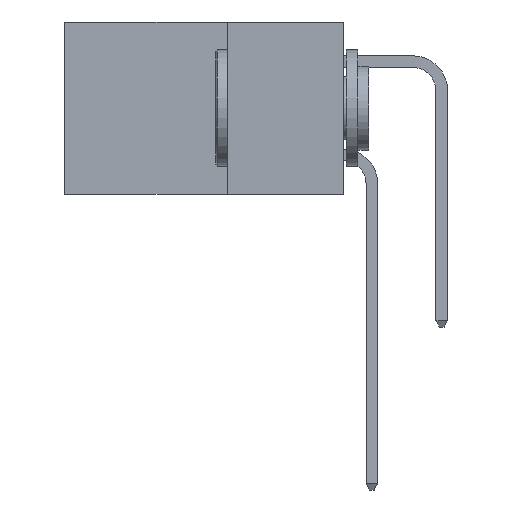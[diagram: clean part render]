
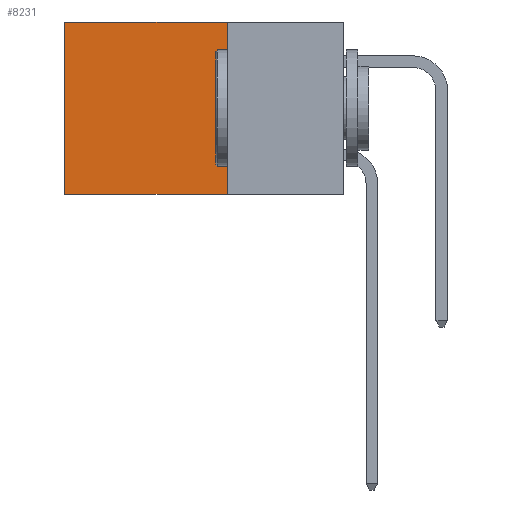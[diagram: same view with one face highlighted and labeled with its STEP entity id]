
A CAD part, left-side view. The second image highlights one B-rep face of the part: STEP entity #8231.
In plain terms, the highlighted planar face has unit normal (-1, 0, 0).
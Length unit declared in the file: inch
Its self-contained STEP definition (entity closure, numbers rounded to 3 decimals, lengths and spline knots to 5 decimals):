
#2493 = VECTOR ( 'NONE', #8146, 39.37008 ) ;
#2675 = EDGE_CURVE ( 'NONE', #8858, #2737, #11368, .T. ) ;
#2737 = VERTEX_POINT ( 'NONE', #3919 ) ;
#3371 = AXIS2_PLACEMENT_3D ( 'NONE', #12109, #11923, #11915 ) ;
#3919 = CARTESIAN_POINT ( 'NONE',  ( 0.2615, 0.6, 0. ) ) ;
#4006 = LINE ( 'NONE', #8329, #12666 ) ;
#4669 = ORIENTED_EDGE ( 'NONE', *, *, #14275, .F. ) ;
#4703 = EDGE_LOOP ( 'NONE', ( #7932, #4669, #14230, #9532 ) ) ;
#4789 = EDGE_CURVE ( 'NONE', #8858, #9702, #7465, .T. ) ;
#4998 = VECTOR ( 'NONE', #6668, 39.37008 ) ;
#5475 = CARTESIAN_POINT ( 'NONE',  ( 0.2615, 0.25, 0. ) ) ;
#5840 = FACE_OUTER_BOUND ( 'NONE', #4703, .T. ) ;
#6668 = DIRECTION ( 'NONE',  ( 0., 1., 0. ) ) ;
#6721 = CARTESIAN_POINT ( 'NONE',  ( 0.2615, 0.25, 0. ) ) ;
#7397 = EDGE_CURVE ( 'NONE', #2737, #14046, #8167, .T. ) ;
#7465 = LINE ( 'NONE', #11857, #9760 ) ;
#7932 = ORIENTED_EDGE ( 'NONE', *, *, #7397, .T. ) ;
#7980 = CARTESIAN_POINT ( 'NONE',  ( 0.2615, 0.6, -0.37 ) ) ;
#8146 = DIRECTION ( 'NONE',  ( 0., 0., -1. ) ) ;
#8167 = LINE ( 'NONE', #7980, #2493 ) ;
#8231 = ADVANCED_FACE ( 'NONE', ( #5840 ), #12163, .F. ) ;
#8278 = DIRECTION ( 'NONE',  ( 0., 1., 0. ) ) ;
#8329 = CARTESIAN_POINT ( 'NONE',  ( 0.2615, 0.25, -0.37 ) ) ;
#8858 = VERTEX_POINT ( 'NONE', #6721 ) ;
#9203 = CARTESIAN_POINT ( 'NONE',  ( 0.2615, 0.25, -0.37 ) ) ;
#9532 = ORIENTED_EDGE ( 'NONE', *, *, #2675, .T. ) ;
#9702 = VERTEX_POINT ( 'NONE', #9203 ) ;
#9760 = VECTOR ( 'NONE', #12223, 39.37008 ) ;
#10356 = CARTESIAN_POINT ( 'NONE',  ( 0.2615, 0.6, -0.37 ) ) ;
#11368 = LINE ( 'NONE', #5475, #4998 ) ;
#11857 = CARTESIAN_POINT ( 'NONE',  ( 0.2615, 0.25, -0.37 ) ) ;
#11915 = DIRECTION ( 'NONE',  ( 0., 0., -1. ) ) ;
#11923 = DIRECTION ( 'NONE',  ( 1., 0., 0. ) ) ;
#12109 = CARTESIAN_POINT ( 'NONE',  ( 0.2615, 0.25, -0.37 ) ) ;
#12163 = PLANE ( 'NONE',  #3371 ) ;
#12223 = DIRECTION ( 'NONE',  ( 0., 0., -1. ) ) ;
#12666 = VECTOR ( 'NONE', #8278, 39.37008 ) ;
#14046 = VERTEX_POINT ( 'NONE', #10356 ) ;
#14230 = ORIENTED_EDGE ( 'NONE', *, *, #4789, .F. ) ;
#14275 = EDGE_CURVE ( 'NONE', #9702, #14046, #4006, .T. ) ;
